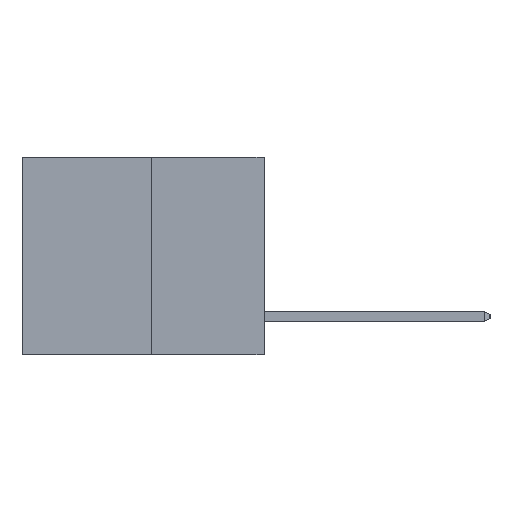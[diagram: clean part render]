
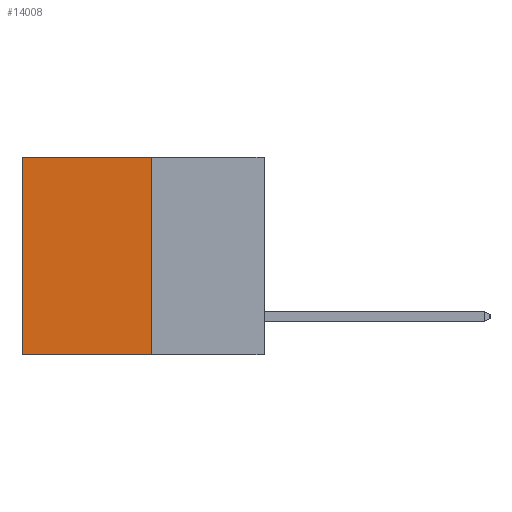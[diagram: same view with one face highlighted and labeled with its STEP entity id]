
A CAD part, left-side view. The second image highlights one B-rep face of the part: STEP entity #14008.
In plain terms, the highlighted planar face has unit normal (-1, 0, 0).
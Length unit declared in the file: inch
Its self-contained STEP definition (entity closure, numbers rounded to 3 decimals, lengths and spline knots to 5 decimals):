
#82 = CARTESIAN_POINT ( 'NONE',  ( 0.3165, 0.6, -0.49 ) ) ;
#196 = ORIENTED_EDGE ( 'NONE', *, *, #9824, .T. ) ;
#286 = VECTOR ( 'NONE', #10357, 39.37008 ) ;
#626 = EDGE_LOOP ( 'NONE', ( #13995, #12880, #8297, #196 ) ) ;
#680 = AXIS2_PLACEMENT_3D ( 'NONE', #5213, #12919, #5062 ) ;
#1342 = VERTEX_POINT ( 'NONE', #2949 ) ;
#2480 = LINE ( 'NONE', #2659, #6000 ) ;
#2503 = EDGE_CURVE ( 'NONE', #7958, #7715, #3119, .T. ) ;
#2659 = CARTESIAN_POINT ( 'NONE',  ( 0.3165, 0.28, -0.49 ) ) ;
#2949 = CARTESIAN_POINT ( 'NONE',  ( 0.3165, 0.28, -0.49 ) ) ;
#3119 = LINE ( 'NONE', #3236, #5404 ) ;
#3151 = DIRECTION ( 'NONE',  ( 0., 0., -1. ) ) ;
#3236 = CARTESIAN_POINT ( 'NONE',  ( 0.3165, 0.6, -0.49 ) ) ;
#4654 = CARTESIAN_POINT ( 'NONE',  ( 0.3165, 0.28, 0. ) ) ;
#4847 = DIRECTION ( 'NONE',  ( 0., 0., -1. ) ) ;
#5062 = DIRECTION ( 'NONE',  ( 0., 0., -1. ) ) ;
#5213 = CARTESIAN_POINT ( 'NONE',  ( 0.3165, 0.28, -0.49 ) ) ;
#5404 = VECTOR ( 'NONE', #3151, 39.37008 ) ;
#6000 = VECTOR ( 'NONE', #4847, 39.37008 ) ;
#6117 = CARTESIAN_POINT ( 'NONE',  ( 0.3165, 0.28, 0. ) ) ;
#6330 = FACE_OUTER_BOUND ( 'NONE', #626, .T. ) ;
#7335 = EDGE_CURVE ( 'NONE', #1342, #7715, #12779, .T. ) ;
#7715 = VERTEX_POINT ( 'NONE', #82 ) ;
#7958 = VERTEX_POINT ( 'NONE', #14017 ) ;
#8297 = ORIENTED_EDGE ( 'NONE', *, *, #13087, .F. ) ;
#9824 = EDGE_CURVE ( 'NONE', #12618, #7958, #11467, .T. ) ;
#10357 = DIRECTION ( 'NONE',  ( 0., 1., 0. ) ) ;
#10839 = PLANE ( 'NONE',  #680 ) ;
#11467 = LINE ( 'NONE', #4654, #12704 ) ;
#11503 = CARTESIAN_POINT ( 'NONE',  ( 0.3165, 0.28, -0.49 ) ) ;
#12618 = VERTEX_POINT ( 'NONE', #6117 ) ;
#12625 = DIRECTION ( 'NONE',  ( 0., 1., 0. ) ) ;
#12704 = VECTOR ( 'NONE', #12625, 39.37008 ) ;
#12779 = LINE ( 'NONE', #11503, #286 ) ;
#12880 = ORIENTED_EDGE ( 'NONE', *, *, #7335, .F. ) ;
#12919 = DIRECTION ( 'NONE',  ( 1., 0., 0. ) ) ;
#13087 = EDGE_CURVE ( 'NONE', #12618, #1342, #2480, .T. ) ;
#13995 = ORIENTED_EDGE ( 'NONE', *, *, #2503, .T. ) ;
#14008 = ADVANCED_FACE ( 'NONE', ( #6330 ), #10839, .F. ) ;
#14017 = CARTESIAN_POINT ( 'NONE',  ( 0.3165, 0.6, 0. ) ) ;
